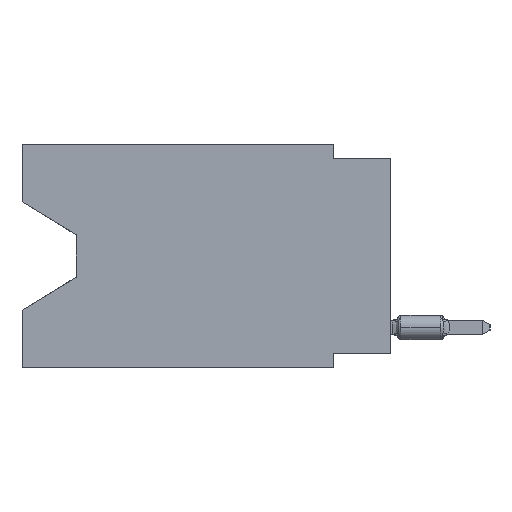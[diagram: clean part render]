
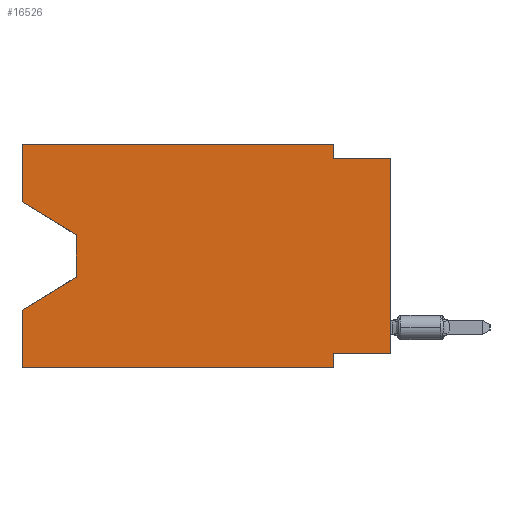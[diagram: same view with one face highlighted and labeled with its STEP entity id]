
A CAD part, left-side view. The second image highlights one B-rep face of the part: STEP entity #16526.
In plain terms, the highlighted planar face has unit normal (-1, 0, 0).
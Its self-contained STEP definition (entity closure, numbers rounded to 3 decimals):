
#926 = ORIENTED_EDGE ( 'NONE', *, *, #36934, .T. ) ;
#949 = CARTESIAN_POINT ( 'NONE',  ( 0., 13.97, -4.013 ) ) ;
#1085 = DIRECTION ( 'NONE',  ( 0., 0., -1. ) ) ;
#1090 = LINE ( 'NONE', #7822, #4720 ) ;
#2122 = EDGE_CURVE ( 'NONE', #17493, #8027, #18040, .T. ) ;
#3618 = DIRECTION ( 'NONE',  ( 1., 0., 0. ) ) ;
#3641 = LINE ( 'NONE', #35799, #26695 ) ;
#4720 = VECTOR ( 'NONE', #33449, 1000. ) ;
#5029 = ORIENTED_EDGE ( 'NONE', *, *, #2122, .F. ) ;
#5327 = ORIENTED_EDGE ( 'NONE', *, *, #15107, .T. ) ;
#5772 = CARTESIAN_POINT ( 'NONE',  ( 0., 13.97, -4.013 ) ) ;
#6268 = CARTESIAN_POINT ( 'NONE',  ( 0., 0., -9.271 ) ) ;
#6462 = LINE ( 'NONE', #41164, #39562 ) ;
#6568 = CARTESIAN_POINT ( 'NONE',  ( 0., 0., 0. ) ) ;
#6953 = EDGE_CURVE ( 'NONE', #8272, #36693, #1090, .T. ) ;
#7026 = VERTEX_POINT ( 'NONE', #11386 ) ;
#7822 = CARTESIAN_POINT ( 'NONE',  ( 0., 16.383, 0. ) ) ;
#7836 = DIRECTION ( 'NONE',  ( 0., 0., -1. ) ) ;
#8027 = VERTEX_POINT ( 'NONE', #23817 ) ;
#8272 = VERTEX_POINT ( 'NONE', #22898 ) ;
#8461 = ORIENTED_EDGE ( 'NONE', *, *, #27861, .F. ) ;
#8863 = LINE ( 'NONE', #41428, #31455 ) ;
#9008 = DIRECTION ( 'NONE',  ( 0., 0., 1. ) ) ;
#9724 = DIRECTION ( 'NONE',  ( 0., 0., 1. ) ) ;
#10298 = VECTOR ( 'NONE', #9724, 1000. ) ;
#11386 = CARTESIAN_POINT ( 'NONE',  ( 0., 0., -0.635 ) ) ;
#13762 = VERTEX_POINT ( 'NONE', #20009 ) ;
#13888 = DIRECTION ( 'NONE',  ( 0., -1., 0. ) ) ;
#14027 = ORIENTED_EDGE ( 'NONE', *, *, #34806, .F. ) ;
#14440 = EDGE_CURVE ( 'NONE', #15831, #17493, #38010, .T. ) ;
#15107 = EDGE_CURVE ( 'NONE', #13762, #15487, #18131, .T. ) ;
#15487 = VERTEX_POINT ( 'NONE', #25716 ) ;
#15831 = VERTEX_POINT ( 'NONE', #24293 ) ;
#16526 = ADVANCED_FACE ( 'NONE', ( #26526 ), #19600, .F. ) ;
#16831 = EDGE_CURVE ( 'NONE', #29045, #36269, #8863, .T. ) ;
#17208 = EDGE_CURVE ( 'NONE', #29045, #8272, #6462, .T. ) ;
#17460 = CARTESIAN_POINT ( 'NONE',  ( 0., 0., -0.635 ) ) ;
#17493 = VERTEX_POINT ( 'NONE', #19881 ) ;
#18025 = VECTOR ( 'NONE', #13888, 1000. ) ;
#18040 = LINE ( 'NONE', #40945, #40710 ) ;
#18131 = LINE ( 'NONE', #24627, #25309 ) ;
#18200 = ORIENTED_EDGE ( 'NONE', *, *, #16831, .T. ) ;
#18733 = DIRECTION ( 'NONE',  ( 0., 0.855, -0.519 ) ) ;
#19040 = LINE ( 'NONE', #28301, #36704 ) ;
#19279 = ORIENTED_EDGE ( 'NONE', *, *, #17208, .F. ) ;
#19600 = PLANE ( 'NONE',  #37484 ) ;
#19612 = EDGE_CURVE ( 'NONE', #36269, #13762, #37519, .T. ) ;
#19746 = CARTESIAN_POINT ( 'NONE',  ( 0., 2.54, -0.635 ) ) ;
#19881 = CARTESIAN_POINT ( 'NONE',  ( 0., 2.54, -9.271 ) ) ;
#20009 = CARTESIAN_POINT ( 'NONE',  ( 0., 13.97, -5.893 ) ) ;
#20026 = VERTEX_POINT ( 'NONE', #21291 ) ;
#21291 = CARTESIAN_POINT ( 'NONE',  ( 0., 16.383, -9.906 ) ) ;
#22370 = DIRECTION ( 'NONE',  ( 0., 0., -1. ) ) ;
#22898 = CARTESIAN_POINT ( 'NONE',  ( 0., 16.383, 0. ) ) ;
#23551 = LINE ( 'NONE', #17460, #18025 ) ;
#23639 = CARTESIAN_POINT ( 'NONE',  ( 0., 16.383, -2.546 ) ) ;
#23817 = CARTESIAN_POINT ( 'NONE',  ( 0., 2.54, -9.906 ) ) ;
#23995 = VECTOR ( 'NONE', #7836, 1000. ) ;
#24293 = CARTESIAN_POINT ( 'NONE',  ( 0., 0., -9.271 ) ) ;
#24627 = CARTESIAN_POINT ( 'NONE',  ( 0., 13.97, -5.893 ) ) ;
#25073 = ORIENTED_EDGE ( 'NONE', *, *, #31101, .F. ) ;
#25164 = DIRECTION ( 'NONE',  ( 0., 0., -1. ) ) ;
#25309 = VECTOR ( 'NONE', #18733, 1000. ) ;
#25716 = CARTESIAN_POINT ( 'NONE',  ( 0., 16.383, -7.36 ) ) ;
#25819 = EDGE_LOOP ( 'NONE', ( #18200, #30781, #5327, #14027, #32123, #5029, #40819, #926, #8461, #25073, #29835, #19279 ) ) ;
#26526 = FACE_OUTER_BOUND ( 'NONE', #25819, .T. ) ;
#26569 = CARTESIAN_POINT ( 'NONE',  ( 0., 2.54, 0. ) ) ;
#26695 = VECTOR ( 'NONE', #36001, 1000. ) ;
#27861 = EDGE_CURVE ( 'NONE', #34350, #7026, #23551, .T. ) ;
#28301 = CARTESIAN_POINT ( 'NONE',  ( 0., 16.383, 0. ) ) ;
#28815 = DIRECTION ( 'NONE',  ( 0., -0.855, -0.519 ) ) ;
#29045 = VERTEX_POINT ( 'NONE', #23639 ) ;
#29292 = VECTOR ( 'NONE', #38838, 1000. ) ;
#29835 = ORIENTED_EDGE ( 'NONE', *, *, #6953, .F. ) ;
#30516 = CARTESIAN_POINT ( 'NONE',  ( 0., 2.54, 0. ) ) ;
#30781 = ORIENTED_EDGE ( 'NONE', *, *, #19612, .T. ) ;
#31054 = EDGE_CURVE ( 'NONE', #20026, #8027, #3641, .T. ) ;
#31101 = EDGE_CURVE ( 'NONE', #36693, #34350, #33461, .T. ) ;
#31455 = VECTOR ( 'NONE', #28815, 1000. ) ;
#31598 = LINE ( 'NONE', #6568, #10298 ) ;
#32123 = ORIENTED_EDGE ( 'NONE', *, *, #31054, .T. ) ;
#32422 = CARTESIAN_POINT ( 'NONE',  ( 0., 16.383, 0. ) ) ;
#33449 = DIRECTION ( 'NONE',  ( 0., -1., 0. ) ) ;
#33461 = LINE ( 'NONE', #30516, #23995 ) ;
#34350 = VERTEX_POINT ( 'NONE', #19746 ) ;
#34806 = EDGE_CURVE ( 'NONE', #20026, #15487, #19040, .T. ) ;
#35799 = CARTESIAN_POINT ( 'NONE',  ( 0., 16.383, -9.906 ) ) ;
#36001 = DIRECTION ( 'NONE',  ( 0., -1., 0. ) ) ;
#36269 = VERTEX_POINT ( 'NONE', #949 ) ;
#36693 = VERTEX_POINT ( 'NONE', #26569 ) ;
#36704 = VECTOR ( 'NONE', #38172, 1000. ) ;
#36934 = EDGE_CURVE ( 'NONE', #15831, #7026, #31598, .T. ) ;
#37484 = AXIS2_PLACEMENT_3D ( 'NONE', #32422, #3618, #1085 ) ;
#37519 = LINE ( 'NONE', #5772, #37778 ) ;
#37778 = VECTOR ( 'NONE', #22370, 1000. ) ;
#38010 = LINE ( 'NONE', #6268, #29292 ) ;
#38172 = DIRECTION ( 'NONE',  ( 0., 0., 1. ) ) ;
#38838 = DIRECTION ( 'NONE',  ( 0., 1., 0. ) ) ;
#39562 = VECTOR ( 'NONE', #9008, 1000. ) ;
#40710 = VECTOR ( 'NONE', #25164, 1000. ) ;
#40819 = ORIENTED_EDGE ( 'NONE', *, *, #14440, .F. ) ;
#40945 = CARTESIAN_POINT ( 'NONE',  ( 0., 2.54, -9.906 ) ) ;
#41164 = CARTESIAN_POINT ( 'NONE',  ( 0., 16.383, 0. ) ) ;
#41428 = CARTESIAN_POINT ( 'NONE',  ( 0., 16.383, -2.546 ) ) ;
